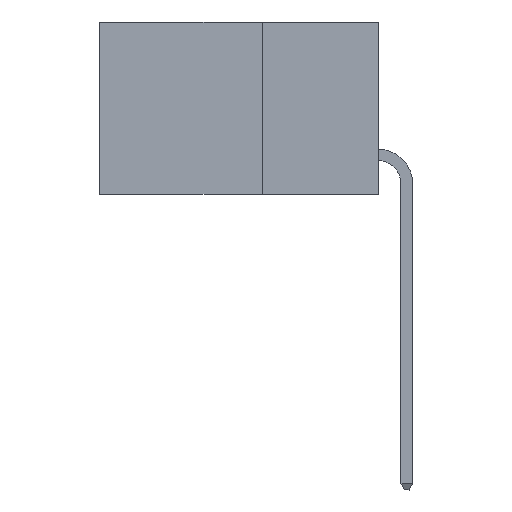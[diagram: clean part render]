
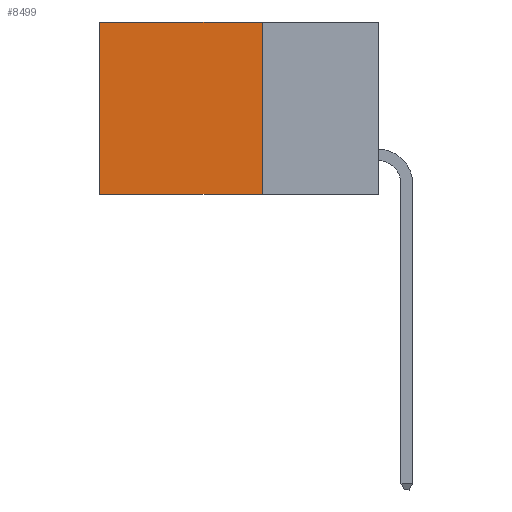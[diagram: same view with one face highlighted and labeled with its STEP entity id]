
A CAD part, left-side view. The second image highlights one B-rep face of the part: STEP entity #8499.
In plain terms, the highlighted planar face has unit normal (-1, 0, 0).
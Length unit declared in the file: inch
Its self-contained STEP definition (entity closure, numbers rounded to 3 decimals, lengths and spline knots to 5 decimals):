
#837 = EDGE_LOOP ( 'NONE', ( #7089, #2637, #2779, #8720 ) ) ;
#979 = CARTESIAN_POINT ( 'NONE',  ( 0.298, 0.25, 0. ) ) ;
#1033 = EDGE_CURVE ( 'NONE', #8837, #2312, #1616, .T. ) ;
#1042 = CARTESIAN_POINT ( 'NONE',  ( 0.298, 0.25, 0. ) ) ;
#1528 = LINE ( 'NONE', #3600, #6235 ) ;
#1616 = LINE ( 'NONE', #8826, #9000 ) ;
#2040 = CARTESIAN_POINT ( 'NONE',  ( 0.298, 0.25, 0. ) ) ;
#2312 = VERTEX_POINT ( 'NONE', #3122 ) ;
#2359 = FACE_OUTER_BOUND ( 'NONE', #837, .T. ) ;
#2637 = ORIENTED_EDGE ( 'NONE', *, *, #1033, .F. ) ;
#2776 = DIRECTION ( 'NONE',  ( 0., 0., -1. ) ) ;
#2779 = ORIENTED_EDGE ( 'NONE', *, *, #8514, .F. ) ;
#3122 = CARTESIAN_POINT ( 'NONE',  ( 0.298, 0.6, -0.37 ) ) ;
#3317 = CARTESIAN_POINT ( 'NONE',  ( 0.298, 0.6, 0. ) ) ;
#3550 = VERTEX_POINT ( 'NONE', #3317 ) ;
#3600 = CARTESIAN_POINT ( 'NONE',  ( 0.298, 0.6, 0. ) ) ;
#4352 = VECTOR ( 'NONE', #4447, 39.37008 ) ;
#4447 = DIRECTION ( 'NONE',  ( 0., 0., -1. ) ) ;
#4843 = AXIS2_PLACEMENT_3D ( 'NONE', #1042, #7648, #2776 ) ;
#5865 = VECTOR ( 'NONE', #10031, 39.37008 ) ;
#6101 = LINE ( 'NONE', #2040, #5865 ) ;
#6235 = VECTOR ( 'NONE', #8424, 39.37008 ) ;
#6272 = EDGE_CURVE ( 'NONE', #7783, #3550, #6101, .T. ) ;
#6721 = LINE ( 'NONE', #8451, #4352 ) ;
#7089 = ORIENTED_EDGE ( 'NONE', *, *, #9595, .T. ) ;
#7331 = CARTESIAN_POINT ( 'NONE',  ( 0.298, 0.25, -0.37 ) ) ;
#7648 = DIRECTION ( 'NONE',  ( 1., 0., 0. ) ) ;
#7783 = VERTEX_POINT ( 'NONE', #979 ) ;
#8424 = DIRECTION ( 'NONE',  ( 0., 0., -1. ) ) ;
#8451 = CARTESIAN_POINT ( 'NONE',  ( 0.298, 0.25, 0. ) ) ;
#8499 = ADVANCED_FACE ( 'NONE', ( #2359 ), #9857, .F. ) ;
#8514 = EDGE_CURVE ( 'NONE', #7783, #8837, #6721, .T. ) ;
#8720 = ORIENTED_EDGE ( 'NONE', *, *, #6272, .T. ) ;
#8826 = CARTESIAN_POINT ( 'NONE',  ( 0.298, 0.25, -0.37 ) ) ;
#8837 = VERTEX_POINT ( 'NONE', #7331 ) ;
#8921 = DIRECTION ( 'NONE',  ( 0., 1., 0. ) ) ;
#9000 = VECTOR ( 'NONE', #8921, 39.37008 ) ;
#9595 = EDGE_CURVE ( 'NONE', #3550, #2312, #1528, .T. ) ;
#9857 = PLANE ( 'NONE',  #4843 ) ;
#10031 = DIRECTION ( 'NONE',  ( 0., 1., 0. ) ) ;
